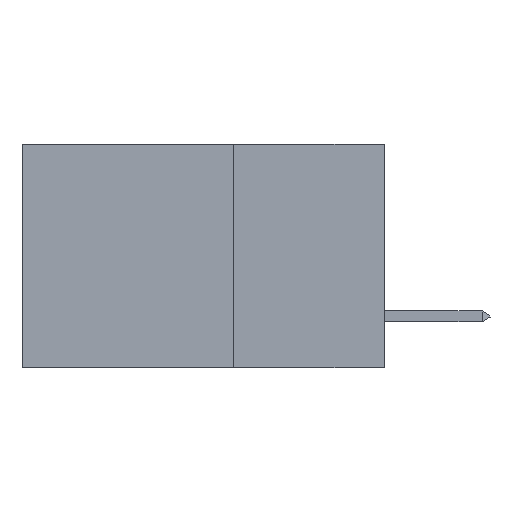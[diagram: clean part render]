
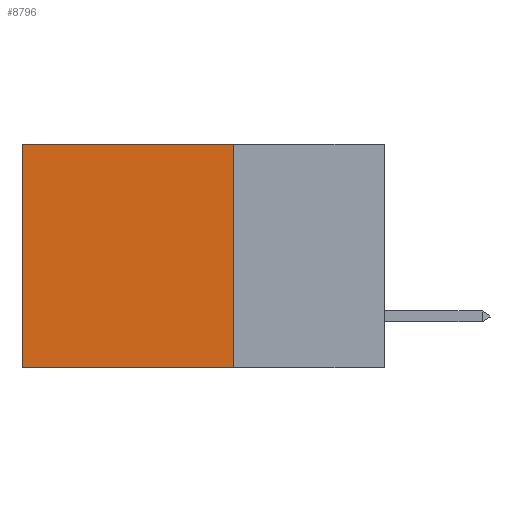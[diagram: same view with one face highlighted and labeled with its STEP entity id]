
A CAD part, left-side view. The second image highlights one B-rep face of the part: STEP entity #8796.
In plain terms, the highlighted planar face has unit normal (-1, 0, 0).
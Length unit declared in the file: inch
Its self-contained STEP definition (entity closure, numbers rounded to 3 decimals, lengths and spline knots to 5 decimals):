
#161 = CARTESIAN_POINT ( 'NONE',  ( 0.2875, 0.6, 0. ) ) ;
#1498 = CARTESIAN_POINT ( 'NONE',  ( 0.2875, 0.6, 0. ) ) ;
#1727 = CARTESIAN_POINT ( 'NONE',  ( 0.2875, 0.6, -0.37 ) ) ;
#2083 = VECTOR ( 'NONE', #21308, 39.37008 ) ;
#2775 = DIRECTION ( 'NONE',  ( 0., 0., -1. ) ) ;
#3621 = LINE ( 'NONE', #1498, #19079 ) ;
#4997 = CARTESIAN_POINT ( 'NONE',  ( 0.2875, 0.25, 0. ) ) ;
#5194 = VECTOR ( 'NONE', #14990, 39.37008 ) ;
#5869 = VECTOR ( 'NONE', #21254, 39.37008 ) ;
#6393 = FACE_OUTER_BOUND ( 'NONE', #6651, .T. ) ;
#6651 = EDGE_LOOP ( 'NONE', ( #24668, #22557, #16440, #13142 ) ) ;
#7080 = EDGE_CURVE ( 'NONE', #17638, #12269, #10008, .T. ) ;
#8738 = VERTEX_POINT ( 'NONE', #1727 ) ;
#8796 = ADVANCED_FACE ( 'NONE', ( #6393 ), #10295, .F. ) ;
#9834 = EDGE_CURVE ( 'NONE', #13505, #8738, #3621, .T. ) ;
#10008 = LINE ( 'NONE', #23281, #2083 ) ;
#10295 = PLANE ( 'NONE',  #16022 ) ;
#10941 = LINE ( 'NONE', #19204, #5869 ) ;
#12165 = LINE ( 'NONE', #4997, #5194 ) ;
#12269 = VERTEX_POINT ( 'NONE', #15034 ) ;
#13142 = ORIENTED_EDGE ( 'NONE', *, *, #24539, .T. ) ;
#13505 = VERTEX_POINT ( 'NONE', #161 ) ;
#14886 = DIRECTION ( 'NONE',  ( 1., 0., 0. ) ) ;
#14990 = DIRECTION ( 'NONE',  ( 0., 1., 0. ) ) ;
#15034 = CARTESIAN_POINT ( 'NONE',  ( 0.2875, 0.25, -0.37 ) ) ;
#16022 = AXIS2_PLACEMENT_3D ( 'NONE', #20521, #14886, #2775 ) ;
#16440 = ORIENTED_EDGE ( 'NONE', *, *, #7080, .F. ) ;
#17445 = EDGE_CURVE ( 'NONE', #12269, #8738, #10941, .T. ) ;
#17638 = VERTEX_POINT ( 'NONE', #25839 ) ;
#19079 = VECTOR ( 'NONE', #19832, 39.37008 ) ;
#19204 = CARTESIAN_POINT ( 'NONE',  ( 0.2875, 0.25, -0.37 ) ) ;
#19832 = DIRECTION ( 'NONE',  ( 0., 0., -1. ) ) ;
#20521 = CARTESIAN_POINT ( 'NONE',  ( 0.2875, 0.25, 0. ) ) ;
#21254 = DIRECTION ( 'NONE',  ( 0., 1., 0. ) ) ;
#21308 = DIRECTION ( 'NONE',  ( 0., 0., -1. ) ) ;
#22557 = ORIENTED_EDGE ( 'NONE', *, *, #17445, .F. ) ;
#23281 = CARTESIAN_POINT ( 'NONE',  ( 0.2875, 0.25, 0. ) ) ;
#24539 = EDGE_CURVE ( 'NONE', #17638, #13505, #12165, .T. ) ;
#24668 = ORIENTED_EDGE ( 'NONE', *, *, #9834, .T. ) ;
#25839 = CARTESIAN_POINT ( 'NONE',  ( 0.2875, 0.25, 0. ) ) ;
